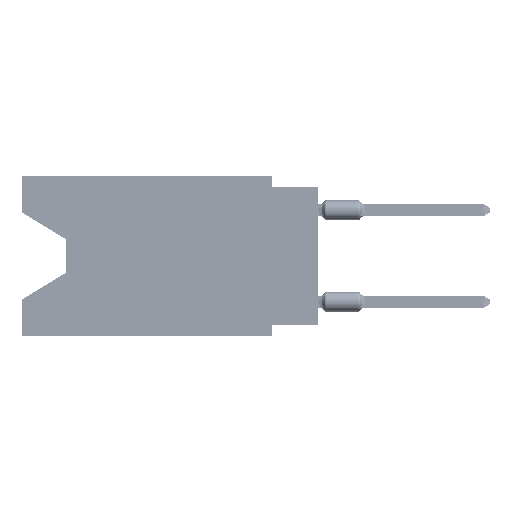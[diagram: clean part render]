
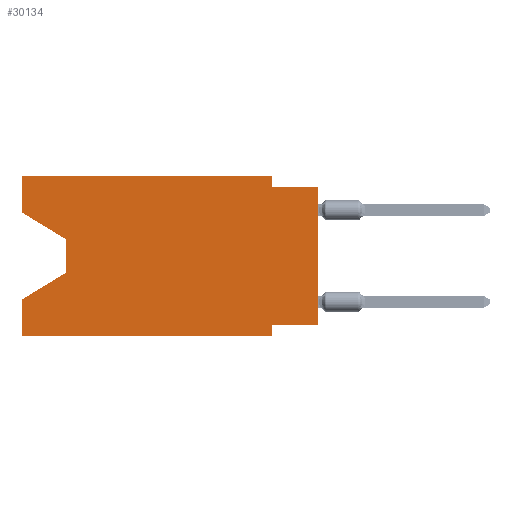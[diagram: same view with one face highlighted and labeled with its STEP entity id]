
A CAD part, left-side view. The second image highlights one B-rep face of the part: STEP entity #30134.
In plain terms, the highlighted planar face has unit normal (-1, 0, 0).
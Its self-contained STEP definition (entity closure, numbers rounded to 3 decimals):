
#438 = VERTEX_POINT ( 'NONE', #55346 ) ;
#983 = VERTEX_POINT ( 'NONE', #34249 ) ;
#4624 = ORIENTED_EDGE ( 'NONE', *, *, #10201, .F. ) ;
#4760 = ORIENTED_EDGE ( 'NONE', *, *, #39791, .T. ) ;
#5149 = DIRECTION ( 'NONE',  ( 0., -1., 0. ) ) ;
#7235 = ORIENTED_EDGE ( 'NONE', *, *, #80791, .T. ) ;
#7701 = VECTOR ( 'NONE', #79671, 1000. ) ;
#9163 = FACE_OUTER_BOUND ( 'NONE', #57396, .T. ) ;
#9236 = CARTESIAN_POINT ( 'NONE',  ( 0., 13.97, -3.505 ) ) ;
#9773 = EDGE_CURVE ( 'NONE', #438, #79638, #26498, .T. ) ;
#10092 = DIRECTION ( 'NONE',  ( 0., 0., -1. ) ) ;
#10201 = EDGE_CURVE ( 'NONE', #43696, #47570, #76506, .T. ) ;
#13134 = DIRECTION ( 'NONE',  ( 0., 0., -1. ) ) ;
#13188 = CARTESIAN_POINT ( 'NONE',  ( 0., 2.54, 0. ) ) ;
#15072 = ORIENTED_EDGE ( 'NONE', *, *, #78433, .T. ) ;
#15266 = CARTESIAN_POINT ( 'NONE',  ( 0., 16.383, 0. ) ) ;
#18525 = VECTOR ( 'NONE', #73423, 1000. ) ;
#19195 = EDGE_CURVE ( 'NONE', #41979, #71883, #33865, .T. ) ;
#19354 = LINE ( 'NONE', #32882, #18525 ) ;
#20632 = DIRECTION ( 'NONE',  ( 0., -1., 0. ) ) ;
#20771 = CARTESIAN_POINT ( 'NONE',  ( 0., 16.383, 0. ) ) ;
#22714 = VECTOR ( 'NONE', #67836, 1000. ) ;
#23800 = VECTOR ( 'NONE', #79328, 1000. ) ;
#25226 = EDGE_CURVE ( 'NONE', #44887, #64531, #85781, .T. ) ;
#25412 = CARTESIAN_POINT ( 'NONE',  ( 0., 0., -8.255 ) ) ;
#25636 = CARTESIAN_POINT ( 'NONE',  ( 0., 0., -0.635 ) ) ;
#26041 = CARTESIAN_POINT ( 'NONE',  ( 0., 0., 0. ) ) ;
#26498 = LINE ( 'NONE', #79246, #49582 ) ;
#27520 = PLANE ( 'NONE',  #40463 ) ;
#27942 = DIRECTION ( 'NONE',  ( 1., 0., 0. ) ) ;
#27951 = CARTESIAN_POINT ( 'NONE',  ( 0., 2.54, -8.89 ) ) ;
#28119 = ORIENTED_EDGE ( 'NONE', *, *, #9773, .T. ) ;
#28595 = ORIENTED_EDGE ( 'NONE', *, *, #38385, .T. ) ;
#28666 = ORIENTED_EDGE ( 'NONE', *, *, #19195, .F. ) ;
#30134 = ADVANCED_FACE ( 'NONE', ( #9163 ), #27520, .F. ) ;
#32162 = VERTEX_POINT ( 'NONE', #84890 ) ;
#32827 = LINE ( 'NONE', #13188, #55288 ) ;
#32882 = CARTESIAN_POINT ( 'NONE',  ( 0., 13.97, -5.385 ) ) ;
#33320 = CARTESIAN_POINT ( 'NONE',  ( 0., 16.383, 0. ) ) ;
#33865 = LINE ( 'NONE', #20771, #58520 ) ;
#34206 = CARTESIAN_POINT ( 'NONE',  ( 0., 0., -0.635 ) ) ;
#34249 = CARTESIAN_POINT ( 'NONE',  ( 0., 16.383, -6.852 ) ) ;
#35768 = DIRECTION ( 'NONE',  ( 0., 0., -1. ) ) ;
#38385 = EDGE_CURVE ( 'NONE', #79638, #57826, #69828, .T. ) ;
#39256 = CARTESIAN_POINT ( 'NONE',  ( 0., 2.54, 0. ) ) ;
#39633 = VECTOR ( 'NONE', #13134, 1000. ) ;
#39791 = EDGE_CURVE ( 'NONE', #32162, #78974, #86019, .T. ) ;
#40463 = AXIS2_PLACEMENT_3D ( 'NONE', #15266, #27942, #35768 ) ;
#41979 = VERTEX_POINT ( 'NONE', #33320 ) ;
#42111 = CARTESIAN_POINT ( 'NONE',  ( 0., 0., -8.255 ) ) ;
#43325 = CARTESIAN_POINT ( 'NONE',  ( 0., 2.54, -0.635 ) ) ;
#43696 = VERTEX_POINT ( 'NONE', #25412 ) ;
#44887 = VERTEX_POINT ( 'NONE', #43325 ) ;
#45294 = CARTESIAN_POINT ( 'NONE',  ( 0., 2.54, -8.255 ) ) ;
#46269 = LINE ( 'NONE', #65026, #39633 ) ;
#46505 = CARTESIAN_POINT ( 'NONE',  ( 0., 13.97, -3.505 ) ) ;
#47469 = CARTESIAN_POINT ( 'NONE',  ( 0., 13.97, -5.385 ) ) ;
#47570 = VERTEX_POINT ( 'NONE', #45294 ) ;
#48144 = VECTOR ( 'NONE', #10092, 1000. ) ;
#48624 = LINE ( 'NONE', #80506, #22714 ) ;
#49582 = VECTOR ( 'NONE', #85355, 1000. ) ;
#49929 = EDGE_CURVE ( 'NONE', #47570, #78974, #46269, .T. ) ;
#52721 = LINE ( 'NONE', #78484, #23800 ) ;
#53057 = LINE ( 'NONE', #26041, #7701 ) ;
#55288 = VECTOR ( 'NONE', #79035, 1000. ) ;
#55346 = CARTESIAN_POINT ( 'NONE',  ( 0., 16.383, -2.038 ) ) ;
#55843 = ORIENTED_EDGE ( 'NONE', *, *, #58992, .F. ) ;
#57396 = EDGE_LOOP ( 'NONE', ( #28119, #28595, #15072, #70783, #4760, #70106, #4624, #7235, #72061, #65399, #28666, #55843 ) ) ;
#57826 = VERTEX_POINT ( 'NONE', #47469 ) ;
#58520 = VECTOR ( 'NONE', #73962, 1000. ) ;
#58992 = EDGE_CURVE ( 'NONE', #438, #41979, #52721, .T. ) ;
#62141 = DIRECTION ( 'NONE',  ( 0., 1., 0. ) ) ;
#64531 = VERTEX_POINT ( 'NONE', #34206 ) ;
#65026 = CARTESIAN_POINT ( 'NONE',  ( 0., 2.54, -8.89 ) ) ;
#65399 = ORIENTED_EDGE ( 'NONE', *, *, #84777, .F. ) ;
#67836 = DIRECTION ( 'NONE',  ( 0., 0., 1. ) ) ;
#69828 = LINE ( 'NONE', #9236, #48144 ) ;
#70106 = ORIENTED_EDGE ( 'NONE', *, *, #49929, .F. ) ;
#70783 = ORIENTED_EDGE ( 'NONE', *, *, #76475, .F. ) ;
#71883 = VERTEX_POINT ( 'NONE', #39256 ) ;
#72061 = ORIENTED_EDGE ( 'NONE', *, *, #25226, .F. ) ;
#72862 = VECTOR ( 'NONE', #5149, 1000. ) ;
#73360 = VECTOR ( 'NONE', #20632, 1000. ) ;
#73423 = DIRECTION ( 'NONE',  ( 0., 0.855, -0.519 ) ) ;
#73962 = DIRECTION ( 'NONE',  ( 0., -1., 0. ) ) ;
#76475 = EDGE_CURVE ( 'NONE', #32162, #983, #48624, .T. ) ;
#76506 = LINE ( 'NONE', #42111, #81485 ) ;
#78433 = EDGE_CURVE ( 'NONE', #57826, #983, #19354, .T. ) ;
#78484 = CARTESIAN_POINT ( 'NONE',  ( 0., 16.383, 0. ) ) ;
#78974 = VERTEX_POINT ( 'NONE', #27951 ) ;
#79035 = DIRECTION ( 'NONE',  ( 0., 0., -1. ) ) ;
#79246 = CARTESIAN_POINT ( 'NONE',  ( 0., 16.383, -2.038 ) ) ;
#79328 = DIRECTION ( 'NONE',  ( 0., 0., 1. ) ) ;
#79638 = VERTEX_POINT ( 'NONE', #46505 ) ;
#79671 = DIRECTION ( 'NONE',  ( 0., 0., 1. ) ) ;
#80371 = CARTESIAN_POINT ( 'NONE',  ( 0., 16.383, -8.89 ) ) ;
#80506 = CARTESIAN_POINT ( 'NONE',  ( 0., 16.383, 0. ) ) ;
#80791 = EDGE_CURVE ( 'NONE', #43696, #64531, #53057, .T. ) ;
#81485 = VECTOR ( 'NONE', #62141, 1000. ) ;
#84777 = EDGE_CURVE ( 'NONE', #71883, #44887, #32827, .T. ) ;
#84890 = CARTESIAN_POINT ( 'NONE',  ( 0., 16.383, -8.89 ) ) ;
#85355 = DIRECTION ( 'NONE',  ( 0., -0.855, -0.519 ) ) ;
#85781 = LINE ( 'NONE', #25636, #72862 ) ;
#86019 = LINE ( 'NONE', #80371, #73360 ) ;
